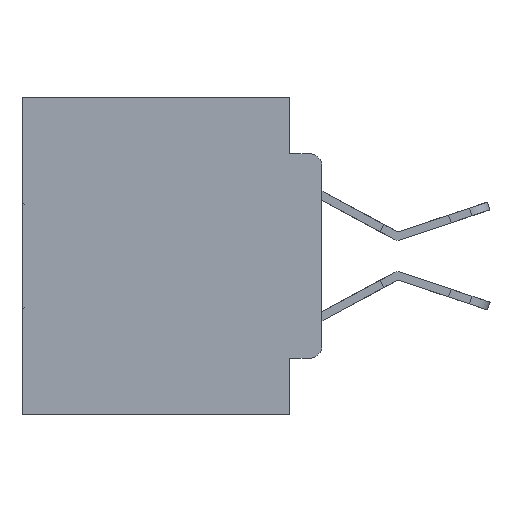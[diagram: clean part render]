
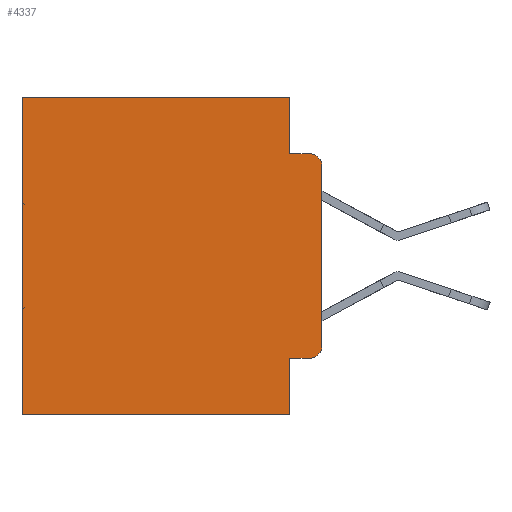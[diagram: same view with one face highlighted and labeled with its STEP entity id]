
A CAD part, left-side view. The second image highlights one B-rep face of the part: STEP entity #4337.
In plain terms, the highlighted planar face has unit normal (-1, 0, 0).
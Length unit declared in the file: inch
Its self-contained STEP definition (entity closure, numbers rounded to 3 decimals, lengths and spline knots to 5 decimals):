
#451 = LINE ( 'NONE', #20978, #4797 ) ;
#469 = EDGE_CURVE ( 'NONE', #6882, #31355, #2721, .T. ) ;
#2639 = DIRECTION ( 'NONE',  ( -1., 0., 0. ) ) ;
#2721 = LINE ( 'NONE', #27752, #3504 ) ;
#2892 = CIRCLE ( 'NONE', #25491, 0.02 ) ;
#3291 = VERTEX_POINT ( 'NONE', #27301 ) ;
#3504 = VECTOR ( 'NONE', #13450, 39.37008 ) ;
#3834 = DIRECTION ( 'NONE',  ( 0., 0., -1. ) ) ;
#4018 = VERTEX_POINT ( 'NONE', #7761 ) ;
#4337 = ADVANCED_FACE ( 'NONE', ( #17459 ), #21472, .F. ) ;
#4797 = VECTOR ( 'NONE', #28489, 39.37008 ) ;
#4914 = LINE ( 'NONE', #14946, #17508 ) ;
#4976 = ORIENTED_EDGE ( 'NONE', *, *, #28888, .T. ) ;
#5964 = AXIS2_PLACEMENT_3D ( 'NONE', #24016, #11483, #29099 ) ;
#6532 = AXIS2_PLACEMENT_3D ( 'NONE', #17705, #2639, #20201 ) ;
#6737 = VECTOR ( 'NONE', #17153, 39.37008 ) ;
#6882 = VERTEX_POINT ( 'NONE', #26840 ) ;
#7761 = CARTESIAN_POINT ( 'NONE',  ( 0.298, 0.02, -0.4115 ) ) ;
#7887 = VERTEX_POINT ( 'NONE', #22328 ) ;
#8199 = EDGE_CURVE ( 'NONE', #6882, #23103, #20262, .T. ) ;
#8505 = EDGE_CURVE ( 'NONE', #29011, #4018, #4914, .T. ) ;
#8784 = ORIENTED_EDGE ( 'NONE', *, *, #13311, .T. ) ;
#9063 = CIRCLE ( 'NONE', #6532, 0.02 ) ;
#9366 = CARTESIAN_POINT ( 'NONE',  ( 0.298, 0.473, 0. ) ) ;
#9598 = CARTESIAN_POINT ( 'NONE',  ( 0.298, 0., -0.1085 ) ) ;
#9742 = CARTESIAN_POINT ( 'NONE',  ( 0.298, 0., -0.3915 ) ) ;
#9844 = LINE ( 'NONE', #19995, #29132 ) ;
#9888 = EDGE_CURVE ( 'NONE', #4018, #30042, #2892, .T. ) ;
#10555 = VERTEX_POINT ( 'NONE', #9598 ) ;
#10902 = EDGE_CURVE ( 'NONE', #10555, #30042, #451, .T. ) ;
#11483 = DIRECTION ( 'NONE',  ( 1., 0., 0. ) ) ;
#12838 = VERTEX_POINT ( 'NONE', #32373 ) ;
#13311 = EDGE_CURVE ( 'NONE', #31355, #7887, #19503, .T. ) ;
#13434 = LINE ( 'NONE', #32200, #6737 ) ;
#13450 = DIRECTION ( 'NONE',  ( 0., 1., 0. ) ) ;
#14484 = DIRECTION ( 'NONE',  ( -1., 0., 0. ) ) ;
#14589 = CARTESIAN_POINT ( 'NONE',  ( 0.298, 0.051, -0.0885 ) ) ;
#14946 = CARTESIAN_POINT ( 'NONE',  ( 0.298, 0.051, -0.4115 ) ) ;
#15482 = EDGE_LOOP ( 'NONE', ( #17253, #4976, #22676, #26867, #18763, #8784, #15847, #18217, #28483, #19788 ) ) ;
#15726 = VECTOR ( 'NONE', #27252, 39.37008 ) ;
#15847 = ORIENTED_EDGE ( 'NONE', *, *, #18393, .F. ) ;
#16369 = CARTESIAN_POINT ( 'NONE',  ( 0.298, 0.051, 0. ) ) ;
#16639 = CARTESIAN_POINT ( 'NONE',  ( 0.298, 0.473, 0. ) ) ;
#17146 = EDGE_CURVE ( 'NONE', #29011, #3291, #29126, .T. ) ;
#17153 = DIRECTION ( 'NONE',  ( 0., 1., 0. ) ) ;
#17253 = ORIENTED_EDGE ( 'NONE', *, *, #10902, .F. ) ;
#17459 = FACE_OUTER_BOUND ( 'NONE', #15482, .T. ) ;
#17508 = VECTOR ( 'NONE', #30006, 39.37008 ) ;
#17705 = CARTESIAN_POINT ( 'NONE',  ( 0.298, 0.02, -0.1085 ) ) ;
#18217 = ORIENTED_EDGE ( 'NONE', *, *, #17146, .F. ) ;
#18393 = EDGE_CURVE ( 'NONE', #3291, #7887, #13434, .T. ) ;
#18763 = ORIENTED_EDGE ( 'NONE', *, *, #469, .T. ) ;
#19261 = DIRECTION ( 'NONE',  ( 0., 0., -1. ) ) ;
#19503 = LINE ( 'NONE', #16639, #32094 ) ;
#19788 = ORIENTED_EDGE ( 'NONE', *, *, #9888, .T. ) ;
#19995 = CARTESIAN_POINT ( 'NONE',  ( 0.298, 0.051, -0.0885 ) ) ;
#20095 = DIRECTION ( 'NONE',  ( 0., -1., 0. ) ) ;
#20201 = DIRECTION ( 'NONE',  ( 0., 0., -1. ) ) ;
#20262 = LINE ( 'NONE', #16369, #25400 ) ;
#20978 = CARTESIAN_POINT ( 'NONE',  ( 0.298, 0., 0. ) ) ;
#21472 = PLANE ( 'NONE',  #5964 ) ;
#22177 = CARTESIAN_POINT ( 'NONE',  ( 0.298, 0.051, 0. ) ) ;
#22328 = CARTESIAN_POINT ( 'NONE',  ( 0.298, 0.473, -0.5 ) ) ;
#22676 = ORIENTED_EDGE ( 'NONE', *, *, #28867, .F. ) ;
#23103 = VERTEX_POINT ( 'NONE', #14589 ) ;
#24016 = CARTESIAN_POINT ( 'NONE',  ( 0.298, 0., 0. ) ) ;
#25400 = VECTOR ( 'NONE', #3834, 39.37008 ) ;
#25491 = AXIS2_PLACEMENT_3D ( 'NONE', #29541, #14484, #32034 ) ;
#25633 = CARTESIAN_POINT ( 'NONE',  ( 0.298, 0.051, -0.4115 ) ) ;
#26840 = CARTESIAN_POINT ( 'NONE',  ( 0.298, 0.051, 0. ) ) ;
#26867 = ORIENTED_EDGE ( 'NONE', *, *, #8199, .F. ) ;
#27252 = DIRECTION ( 'NONE',  ( 0., 0., -1. ) ) ;
#27301 = CARTESIAN_POINT ( 'NONE',  ( 0.298, 0.051, -0.5 ) ) ;
#27752 = CARTESIAN_POINT ( 'NONE',  ( 0.298, 0., 0. ) ) ;
#28483 = ORIENTED_EDGE ( 'NONE', *, *, #8505, .T. ) ;
#28489 = DIRECTION ( 'NONE',  ( 0., 0., -1. ) ) ;
#28867 = EDGE_CURVE ( 'NONE', #23103, #12838, #9844, .T. ) ;
#28888 = EDGE_CURVE ( 'NONE', #10555, #12838, #9063, .T. ) ;
#29011 = VERTEX_POINT ( 'NONE', #25633 ) ;
#29099 = DIRECTION ( 'NONE',  ( 0., 0., -1. ) ) ;
#29126 = LINE ( 'NONE', #22177, #15726 ) ;
#29132 = VECTOR ( 'NONE', #20095, 39.37008 ) ;
#29541 = CARTESIAN_POINT ( 'NONE',  ( 0.298, 0.02, -0.3915 ) ) ;
#30006 = DIRECTION ( 'NONE',  ( 0., -1., 0. ) ) ;
#30042 = VERTEX_POINT ( 'NONE', #9742 ) ;
#31355 = VERTEX_POINT ( 'NONE', #9366 ) ;
#32034 = DIRECTION ( 'NONE',  ( 0., 0., -1. ) ) ;
#32094 = VECTOR ( 'NONE', #19261, 39.37008 ) ;
#32200 = CARTESIAN_POINT ( 'NONE',  ( 0.298, 0., -0.5 ) ) ;
#32373 = CARTESIAN_POINT ( 'NONE',  ( 0.298, 0.02, -0.0885 ) ) ;
